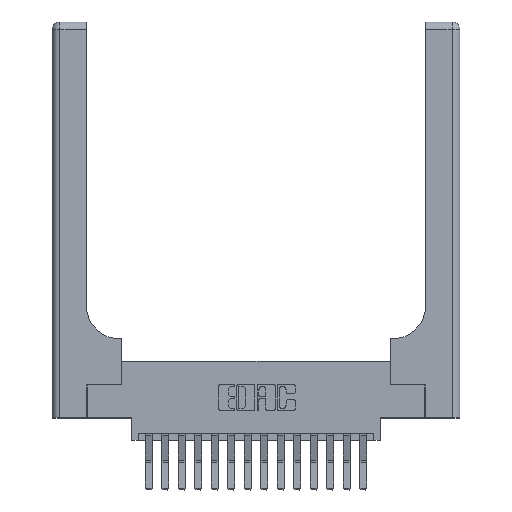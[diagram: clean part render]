
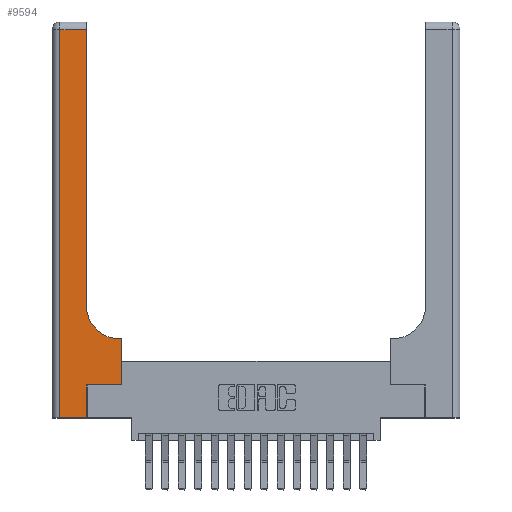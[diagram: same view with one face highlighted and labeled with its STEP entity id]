
A CAD part, top view. The second image highlights one B-rep face of the part: STEP entity #9594.
In plain terms, the highlighted planar face has unit normal (0, 0, 1).
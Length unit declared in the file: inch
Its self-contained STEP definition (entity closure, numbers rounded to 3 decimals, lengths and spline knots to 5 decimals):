
#26 = CARTESIAN_POINT ( 'NONE',  ( 0.26, 0.85, 0.37 ) ) ;
#83 = DIRECTION ( 'NONE',  ( 1., 0., 0. ) ) ;
#258 = CARTESIAN_POINT ( 'NONE',  ( 0.265, 0.25, 0.37 ) ) ;
#742 = VERTEX_POINT ( 'NONE', #16778 ) ;
#1317 = CARTESIAN_POINT ( 'NONE',  ( 0.06, 0., 0.37 ) ) ;
#1331 = CARTESIAN_POINT ( 'NONE',  ( 0., 0., 0.37 ) ) ;
#1381 = DIRECTION ( 'NONE',  ( 0., 1., 0. ) ) ;
#1408 = DIRECTION ( 'NONE',  ( 1., 0., 0. ) ) ;
#1653 = VECTOR ( 'NONE', #13174, 39.37008 ) ;
#1753 = CARTESIAN_POINT ( 'NONE',  ( 0.51, 0.85, 0.37 ) ) ;
#2118 = LINE ( 'NONE', #10968, #8873 ) ;
#2160 = PLANE ( 'NONE',  #13999 ) ;
#2463 = VECTOR ( 'NONE', #83, 39.37008 ) ;
#2782 = LINE ( 'NONE', #4306, #9498 ) ;
#2869 = CARTESIAN_POINT ( 'NONE',  ( 0.26, 3., 0.37 ) ) ;
#3129 = CARTESIAN_POINT ( 'NONE',  ( 0.265, 0., 0.37 ) ) ;
#3324 = DIRECTION ( 'NONE',  ( -1., 0., 0. ) ) ;
#3900 = EDGE_CURVE ( 'NONE', #7370, #14262, #2118, .T. ) ;
#4257 = DIRECTION ( 'NONE',  ( 0., 1., 0. ) ) ;
#4306 = CARTESIAN_POINT ( 'NONE',  ( 0.528, 0.25, 0.37 ) ) ;
#4347 = VECTOR ( 'NONE', #8661, 39.37008 ) ;
#4441 = VERTEX_POINT ( 'NONE', #14510 ) ;
#4592 = ORIENTED_EDGE ( 'NONE', *, *, #9371, .T. ) ;
#4714 = LINE ( 'NONE', #8898, #1653 ) ;
#4730 = ORIENTED_EDGE ( 'NONE', *, *, #7428, .T. ) ;
#4812 = DIRECTION ( 'NONE',  ( -1., 0., 0. ) ) ;
#5045 = ORIENTED_EDGE ( 'NONE', *, *, #6650, .T. ) ;
#5951 = LINE ( 'NONE', #1331, #2463 ) ;
#6204 = EDGE_CURVE ( 'NONE', #9487, #16314, #15239, .T. ) ;
#6261 = CARTESIAN_POINT ( 'NONE',  ( 0., 2.94, 0.37 ) ) ;
#6419 = FACE_OUTER_BOUND ( 'NONE', #10908, .T. ) ;
#6650 = EDGE_CURVE ( 'NONE', #16314, #742, #17303, .T. ) ;
#7039 = AXIS2_PLACEMENT_3D ( 'NONE', #1753, #18086, #16273 ) ;
#7370 = VERTEX_POINT ( 'NONE', #14132 ) ;
#7428 = EDGE_CURVE ( 'NONE', #7482, #9487, #4714, .T. ) ;
#7482 = VERTEX_POINT ( 'NONE', #10529 ) ;
#8661 = DIRECTION ( 'NONE',  ( 0., 1., 0. ) ) ;
#8749 = CARTESIAN_POINT ( 'NONE',  ( 0.528, 0.25, 0.37 ) ) ;
#8873 = VECTOR ( 'NONE', #14073, 39.37008 ) ;
#8898 = CARTESIAN_POINT ( 'NONE',  ( 0.26, 0.6, 0.37 ) ) ;
#9093 = CARTESIAN_POINT ( 'NONE',  ( 0.51, 0.6, 0.37 ) ) ;
#9371 = EDGE_CURVE ( 'NONE', #14262, #10161, #5951, .T. ) ;
#9487 = VERTEX_POINT ( 'NONE', #9093 ) ;
#9498 = VECTOR ( 'NONE', #1381, 39.37008 ) ;
#9594 = ADVANCED_FACE ( 'NONE', ( #6419 ), #2160, .F. ) ;
#10132 = ORIENTED_EDGE ( 'NONE', *, *, #11564, .T. ) ;
#10161 = VERTEX_POINT ( 'NONE', #3129 ) ;
#10463 = VECTOR ( 'NONE', #3324, 39.37008 ) ;
#10529 = CARTESIAN_POINT ( 'NONE',  ( 0.528, 0.6, 0.37 ) ) ;
#10908 = EDGE_LOOP ( 'NONE', ( #5045, #11140, #16602, #4592, #11375, #15205, #10132, #4730, #11032 ) ) ;
#10968 = CARTESIAN_POINT ( 'NONE',  ( 0.06, 3., 0.37 ) ) ;
#11032 = ORIENTED_EDGE ( 'NONE', *, *, #6204, .T. ) ;
#11140 = ORIENTED_EDGE ( 'NONE', *, *, #15443, .T. ) ;
#11375 = ORIENTED_EDGE ( 'NONE', *, *, #13785, .T. ) ;
#11564 = EDGE_CURVE ( 'NONE', #15272, #7482, #2782, .T. ) ;
#11693 = CARTESIAN_POINT ( 'NONE',  ( 0.265, 0., 0.37 ) ) ;
#13065 = LINE ( 'NONE', #258, #15669 ) ;
#13174 = DIRECTION ( 'NONE',  ( -1., 0., 0. ) ) ;
#13785 = EDGE_CURVE ( 'NONE', #10161, #4441, #18696, .T. ) ;
#13999 = AXIS2_PLACEMENT_3D ( 'NONE', #18020, #17825, #4812 ) ;
#14073 = DIRECTION ( 'NONE',  ( 0., -1., 0. ) ) ;
#14132 = CARTESIAN_POINT ( 'NONE',  ( 0.06, 2.94, 0.37 ) ) ;
#14262 = VERTEX_POINT ( 'NONE', #1317 ) ;
#14510 = CARTESIAN_POINT ( 'NONE',  ( 0.265, 0.25, 0.37 ) ) ;
#15007 = LINE ( 'NONE', #6261, #10463 ) ;
#15205 = ORIENTED_EDGE ( 'NONE', *, *, #17894, .T. ) ;
#15239 = CIRCLE ( 'NONE', #7039, 0.25 ) ;
#15272 = VERTEX_POINT ( 'NONE', #8749 ) ;
#15443 = EDGE_CURVE ( 'NONE', #742, #7370, #15007, .T. ) ;
#15669 = VECTOR ( 'NONE', #1408, 39.37008 ) ;
#16273 = DIRECTION ( 'NONE',  ( 1., 0., 0. ) ) ;
#16314 = VERTEX_POINT ( 'NONE', #26 ) ;
#16602 = ORIENTED_EDGE ( 'NONE', *, *, #3900, .T. ) ;
#16778 = CARTESIAN_POINT ( 'NONE',  ( 0.26, 2.94, 0.37 ) ) ;
#17303 = LINE ( 'NONE', #2869, #4347 ) ;
#17825 = DIRECTION ( 'NONE',  ( 0., 0., -1. ) ) ;
#17894 = EDGE_CURVE ( 'NONE', #4441, #15272, #13065, .T. ) ;
#17998 = VECTOR ( 'NONE', #4257, 39.37008 ) ;
#18020 = CARTESIAN_POINT ( 'NONE',  ( 0., 3., 0.37 ) ) ;
#18086 = DIRECTION ( 'NONE',  ( 0., 0., -1. ) ) ;
#18696 = LINE ( 'NONE', #11693, #17998 ) ;
